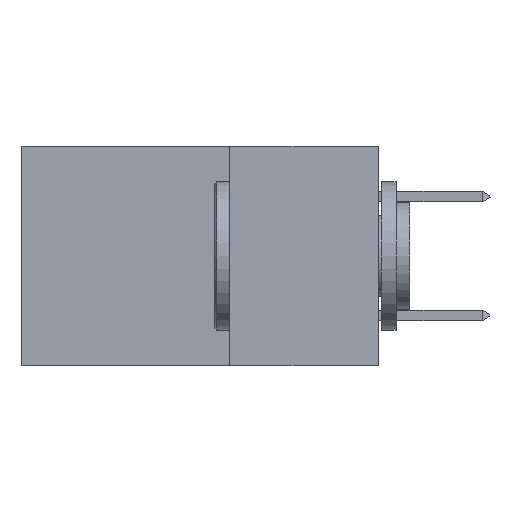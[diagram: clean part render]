
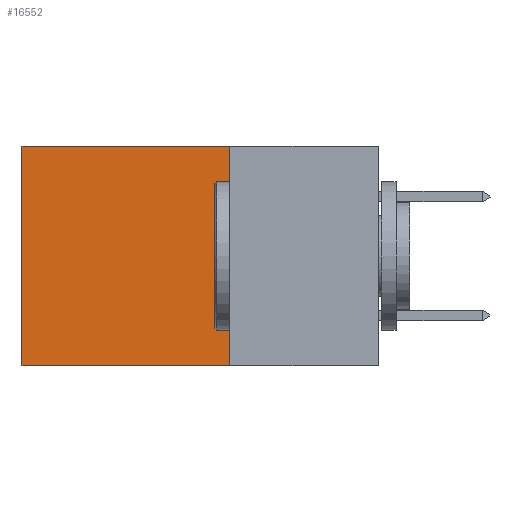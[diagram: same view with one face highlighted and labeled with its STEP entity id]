
A CAD part, left-side view. The second image highlights one B-rep face of the part: STEP entity #16552.
In plain terms, the highlighted planar face has unit normal (-1, 0, 0).
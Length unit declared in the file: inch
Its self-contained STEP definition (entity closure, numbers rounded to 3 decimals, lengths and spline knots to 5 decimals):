
#551 = LINE ( 'NONE', #10502, #20873 ) ;
#1170 = DIRECTION ( 'NONE',  ( 0., 0., -1. ) ) ;
#1369 = CARTESIAN_POINT ( 'NONE',  ( 0.298, 0.6, 0. ) ) ;
#3275 = LINE ( 'NONE', #31085, #21932 ) ;
#4153 = VERTEX_POINT ( 'NONE', #17573 ) ;
#4403 = VERTEX_POINT ( 'NONE', #4986 ) ;
#4986 = CARTESIAN_POINT ( 'NONE',  ( 0.298, 0.6, -0.37 ) ) ;
#7320 = EDGE_LOOP ( 'NONE', ( #24085, #17207, #22756, #24937 ) ) ;
#8208 = AXIS2_PLACEMENT_3D ( 'NONE', #28920, #16384, #1170 ) ;
#8501 = EDGE_CURVE ( 'NONE', #14291, #4403, #551, .T. ) ;
#9935 = LINE ( 'NONE', #29820, #22622 ) ;
#10502 = CARTESIAN_POINT ( 'NONE',  ( 0.298, 0.25, -0.37 ) ) ;
#11087 = DIRECTION ( 'NONE',  ( 0., 1., 0. ) ) ;
#13856 = PLANE ( 'NONE',  #8208 ) ;
#14291 = VERTEX_POINT ( 'NONE', #28269 ) ;
#16193 = CARTESIAN_POINT ( 'NONE',  ( 0.298, 0.25, 0. ) ) ;
#16384 = DIRECTION ( 'NONE',  ( 1., 0., 0. ) ) ;
#16552 = ADVANCED_FACE ( 'NONE', ( #21709 ), #13856, .F. ) ;
#17207 = ORIENTED_EDGE ( 'NONE', *, *, #8501, .F. ) ;
#17573 = CARTESIAN_POINT ( 'NONE',  ( 0.298, 0.6, 0. ) ) ;
#19480 = LINE ( 'NONE', #1369, #25376 ) ;
#20257 = EDGE_CURVE ( 'NONE', #4153, #4403, #19480, .T. ) ;
#20873 = VECTOR ( 'NONE', #28100, 39.37008 ) ;
#21045 = EDGE_CURVE ( 'NONE', #31445, #14291, #9935, .T. ) ;
#21709 = FACE_OUTER_BOUND ( 'NONE', #7320, .T. ) ;
#21932 = VECTOR ( 'NONE', #11087, 39.37008 ) ;
#22622 = VECTOR ( 'NONE', #32322, 39.37008 ) ;
#22756 = ORIENTED_EDGE ( 'NONE', *, *, #21045, .F. ) ;
#24085 = ORIENTED_EDGE ( 'NONE', *, *, #20257, .T. ) ;
#24937 = ORIENTED_EDGE ( 'NONE', *, *, #25142, .T. ) ;
#25142 = EDGE_CURVE ( 'NONE', #31445, #4153, #3275, .T. ) ;
#25376 = VECTOR ( 'NONE', #26720, 39.37008 ) ;
#26720 = DIRECTION ( 'NONE',  ( 0., 0., -1. ) ) ;
#28100 = DIRECTION ( 'NONE',  ( 0., 1., 0. ) ) ;
#28269 = CARTESIAN_POINT ( 'NONE',  ( 0.298, 0.25, -0.37 ) ) ;
#28920 = CARTESIAN_POINT ( 'NONE',  ( 0.298, 0.25, 0. ) ) ;
#29820 = CARTESIAN_POINT ( 'NONE',  ( 0.298, 0.25, 0. ) ) ;
#31085 = CARTESIAN_POINT ( 'NONE',  ( 0.298, 0.25, 0. ) ) ;
#31445 = VERTEX_POINT ( 'NONE', #16193 ) ;
#32322 = DIRECTION ( 'NONE',  ( 0., 0., -1. ) ) ;
